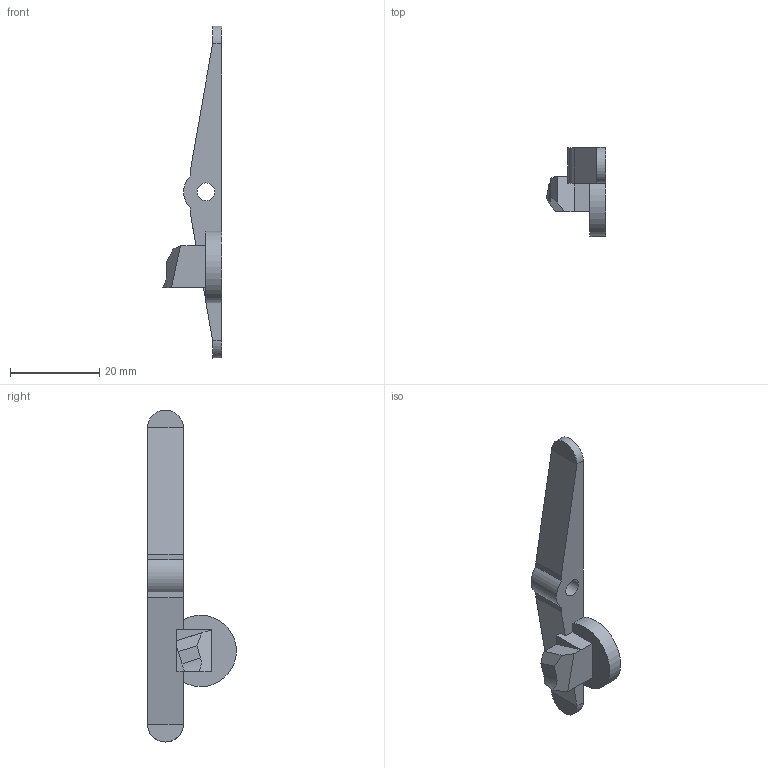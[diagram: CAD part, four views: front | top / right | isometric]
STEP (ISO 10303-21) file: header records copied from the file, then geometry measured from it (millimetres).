
FILE_DESCRIPTION (( 'STEP AP214' ), '1' );
FILE_NAME ('Mag_Release_Right_V0.2A.STEP', '2016-02-15T23:16:34', ( 'WarFairy' ), ( '' ), 'SwSTEP 2.0', 'SolidWorks 2015', '' );
FILE_SCHEMA (( 'AUTOMOTIVE_DESIGN' ));
Length unit declared in the file: millimetre
Products named in the file (1): Mag_Release_Right_V0.2A
Bounding box: 13.25 x 19.91 x 74.4 mm (x, y, z)
Volume: 3719.8 mm3; surface area: 2580.3 mm2
Topology: 1 solids, 1 shells, 29 faces, 77 edges, 50 vertices
Faces by surface type: plane 23, cylinder 6
Full cylindrical faces by diameter (mm): 4 x1
Entity records: 923 total; most frequent: CARTESIAN_POINT 165, ORIENTED_EDGE 152, DIRECTION 144, EDGE_CURVE 76, VECTOR 62, LINE 62, VERTEX_POINT 50, AXIS2_PLACEMENT_3D 41
